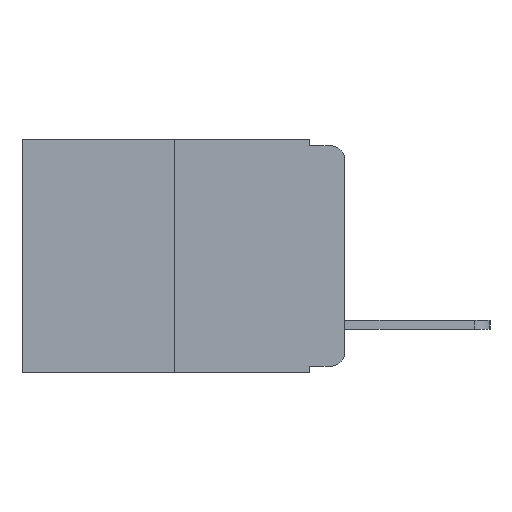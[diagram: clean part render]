
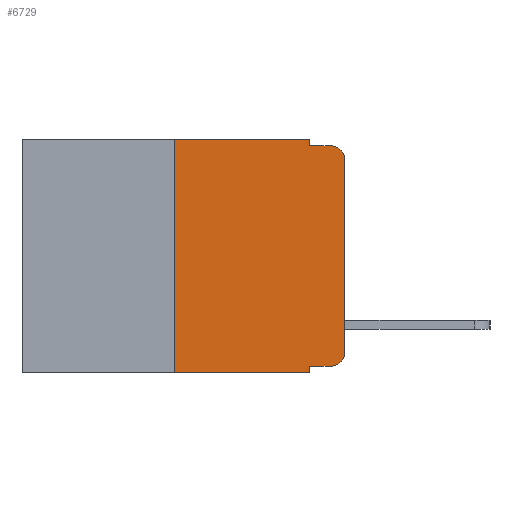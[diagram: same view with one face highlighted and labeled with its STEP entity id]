
A CAD part, left-side view. The second image highlights one B-rep face of the part: STEP entity #6729.
In plain terms, the highlighted planar face has unit normal (-1, 0, 0).
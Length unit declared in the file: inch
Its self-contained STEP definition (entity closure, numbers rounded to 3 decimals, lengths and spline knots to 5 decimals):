
#151 = EDGE_CURVE ( 'NONE', #7042, #2297, #15423, .T. ) ;
#232 = LINE ( 'NONE', #15882, #8161 ) ;
#581 = AXIS2_PLACEMENT_3D ( 'NONE', #13433, #13594, #13365 ) ;
#654 = CARTESIAN_POINT ( 'NONE',  ( 0., 0.25, 0. ) ) ;
#796 = VERTEX_POINT ( 'NONE', #16850 ) ;
#1742 = CARTESIAN_POINT ( 'NONE',  ( 0., 0., -0.03 ) ) ;
#1946 = EDGE_CURVE ( 'NONE', #8417, #2297, #12460, .T. ) ;
#2257 = ORIENTED_EDGE ( 'NONE', *, *, #11082, .T. ) ;
#2287 = CARTESIAN_POINT ( 'NONE',  ( 0., 0.25, -0.343 ) ) ;
#2297 = VERTEX_POINT ( 'NONE', #10767 ) ;
#2502 = ORIENTED_EDGE ( 'NONE', *, *, #1946, .F. ) ;
#2918 = EDGE_CURVE ( 'NONE', #5547, #9491, #232, .T. ) ;
#3244 = ORIENTED_EDGE ( 'NONE', *, *, #15910, .F. ) ;
#3447 = EDGE_CURVE ( 'NONE', #16118, #8417, #16820, .T. ) ;
#4156 = EDGE_CURVE ( 'NONE', #9939, #7042, #15141, .T. ) ;
#5456 = LINE ( 'NONE', #8013, #15496 ) ;
#5547 = VERTEX_POINT ( 'NONE', #2287 ) ;
#5621 = DIRECTION ( 'NONE',  ( 0., 0., -1. ) ) ;
#5883 = CARTESIAN_POINT ( 'NONE',  ( 0., 0.051, 0. ) ) ;
#6541 = AXIS2_PLACEMENT_3D ( 'NONE', #12669, #16809, #13804 ) ;
#6729 = ADVANCED_FACE ( 'NONE', ( #16722 ), #14079, .F. ) ;
#6735 = EDGE_LOOP ( 'NONE', ( #13747, #10405, #2502, #10007, #15934, #3244, #6873, #16375, #2257, #13201 ) ) ;
#6873 = ORIENTED_EDGE ( 'NONE', *, *, #2918, .T. ) ;
#7042 = VERTEX_POINT ( 'NONE', #1742 ) ;
#7877 = DIRECTION ( 'NONE',  ( 0., -1., 0. ) ) ;
#8013 = CARTESIAN_POINT ( 'NONE',  ( 0., 0.473, 0. ) ) ;
#8161 = VECTOR ( 'NONE', #13793, 39.37008 ) ;
#8417 = VERTEX_POINT ( 'NONE', #11287 ) ;
#8789 = CARTESIAN_POINT ( 'NONE',  ( 0., 0., 0. ) ) ;
#8989 = LINE ( 'NONE', #14045, #15505 ) ;
#9220 = VERTEX_POINT ( 'NONE', #654 ) ;
#9491 = VERTEX_POINT ( 'NONE', #12767 ) ;
#9939 = VERTEX_POINT ( 'NONE', #12499 ) ;
#9976 = DIRECTION ( 'NONE',  ( 0., -1., 0. ) ) ;
#10007 = ORIENTED_EDGE ( 'NONE', *, *, #3447, .F. ) ;
#10133 = CARTESIAN_POINT ( 'NONE',  ( 0., 0.051, -0.333 ) ) ;
#10228 = CARTESIAN_POINT ( 'NONE',  ( 0., 0.02, -0.333 ) ) ;
#10405 = ORIENTED_EDGE ( 'NONE', *, *, #151, .T. ) ;
#10767 = CARTESIAN_POINT ( 'NONE',  ( 0., 0.02, -0.01 ) ) ;
#10813 = DIRECTION ( 'NONE',  ( 0., -1., 0. ) ) ;
#11053 = DIRECTION ( 'NONE',  ( 0., 0., -1. ) ) ;
#11077 = VERTEX_POINT ( 'NONE', #10228 ) ;
#11082 = EDGE_CURVE ( 'NONE', #796, #11077, #17294, .T. ) ;
#11133 = DIRECTION ( 'NONE',  ( -1., 0., 0. ) ) ;
#11287 = CARTESIAN_POINT ( 'NONE',  ( 0., 0.051, -0.01 ) ) ;
#11298 = CARTESIAN_POINT ( 'NONE',  ( 0., 0.02, -0.313 ) ) ;
#11671 = VECTOR ( 'NONE', #10813, 39.37008 ) ;
#11936 = VECTOR ( 'NONE', #14368, 39.37008 ) ;
#12460 = LINE ( 'NONE', #15433, #11671 ) ;
#12492 = EDGE_CURVE ( 'NONE', #11077, #9939, #15611, .T. ) ;
#12499 = CARTESIAN_POINT ( 'NONE',  ( 0., 0., -0.313 ) ) ;
#12669 = CARTESIAN_POINT ( 'NONE',  ( 0., 0.02, -0.03 ) ) ;
#12767 = CARTESIAN_POINT ( 'NONE',  ( 0., 0.051, -0.343 ) ) ;
#13194 = AXIS2_PLACEMENT_3D ( 'NONE', #11298, #11133, #11053 ) ;
#13201 = ORIENTED_EDGE ( 'NONE', *, *, #12492, .T. ) ;
#13219 = LINE ( 'NONE', #15156, #15806 ) ;
#13365 = DIRECTION ( 'NONE',  ( 0., 0., -1. ) ) ;
#13433 = CARTESIAN_POINT ( 'NONE',  ( 0., 0.473, 0. ) ) ;
#13445 = CARTESIAN_POINT ( 'NONE',  ( 0., 0.051, 0. ) ) ;
#13594 = DIRECTION ( 'NONE',  ( 1., 0., 0. ) ) ;
#13747 = ORIENTED_EDGE ( 'NONE', *, *, #4156, .T. ) ;
#13793 = DIRECTION ( 'NONE',  ( 0., -1., 0. ) ) ;
#13804 = DIRECTION ( 'NONE',  ( 0., 0., -1. ) ) ;
#13974 = DIRECTION ( 'NONE',  ( 0., 0., -1. ) ) ;
#14045 = CARTESIAN_POINT ( 'NONE',  ( 0., 0.051, 0. ) ) ;
#14079 = PLANE ( 'NONE',  #581 ) ;
#14334 = VECTOR ( 'NONE', #9976, 39.37008 ) ;
#14368 = DIRECTION ( 'NONE',  ( 0., 0., 1. ) ) ;
#14983 = DIRECTION ( 'NONE',  ( 0., 0., 1. ) ) ;
#15141 = LINE ( 'NONE', #8789, #11936 ) ;
#15156 = CARTESIAN_POINT ( 'NONE',  ( 0., 0.25, 0. ) ) ;
#15423 = CIRCLE ( 'NONE', #6541, 0.02 ) ;
#15433 = CARTESIAN_POINT ( 'NONE',  ( 0., 0.051, -0.01 ) ) ;
#15496 = VECTOR ( 'NONE', #7877, 39.37008 ) ;
#15505 = VECTOR ( 'NONE', #13974, 39.37008 ) ;
#15611 = CIRCLE ( 'NONE', #13194, 0.02 ) ;
#15806 = VECTOR ( 'NONE', #14983, 39.37008 ) ;
#15882 = CARTESIAN_POINT ( 'NONE',  ( 0., 0.473, -0.343 ) ) ;
#15910 = EDGE_CURVE ( 'NONE', #5547, #9220, #13219, .T. ) ;
#15934 = ORIENTED_EDGE ( 'NONE', *, *, #17319, .F. ) ;
#16002 = EDGE_CURVE ( 'NONE', #796, #9491, #8989, .T. ) ;
#16118 = VERTEX_POINT ( 'NONE', #13445 ) ;
#16375 = ORIENTED_EDGE ( 'NONE', *, *, #16002, .F. ) ;
#16510 = VECTOR ( 'NONE', #5621, 39.37008 ) ;
#16722 = FACE_OUTER_BOUND ( 'NONE', #6735, .T. ) ;
#16809 = DIRECTION ( 'NONE',  ( -1., 0., 0. ) ) ;
#16820 = LINE ( 'NONE', #5883, #16510 ) ;
#16850 = CARTESIAN_POINT ( 'NONE',  ( 0., 0.051, -0.333 ) ) ;
#17294 = LINE ( 'NONE', #10133, #14334 ) ;
#17319 = EDGE_CURVE ( 'NONE', #9220, #16118, #5456, .T. ) ;
